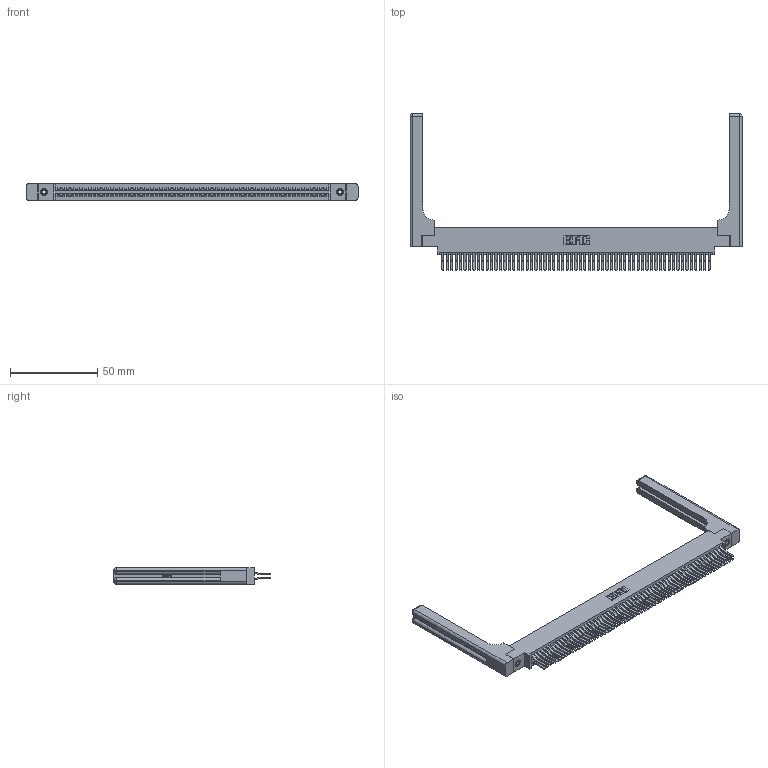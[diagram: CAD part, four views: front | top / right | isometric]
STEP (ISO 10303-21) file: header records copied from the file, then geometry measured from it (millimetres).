
FILE_DESCRIPTION (( 'STEP AP203' ), '1' );
FILE_NAME ('395-122-560-858.STEP', '2019-10-28T09:59:10', ( '' ), ( '' ), 'SwSTEP 2.0', 'SolidWorks 2016', '' );
FILE_SCHEMA (( 'CONFIG_CONTROL_DESIGN' ));
Length unit declared in the file: inch
Products named in the file (5): 345 Part_0.170 Offset - 0.156 Dia-TH; 345-292-001_560 Tail; 345-250-001_345-250-001-102; 345-220-058_345-220-058; 395-122-560-858
Assembly tree (127 placements, depth 2):
  395-122-560-858
    345 Part_0.170 Offset - 0.156 Dia-TH
    345-292-001_560 Tail  x122
    345-250-001_345-250-001-102  x2
    345-220-058_345-220-058  x2
Bounding box: 189.97 x 89.72 x 9.4 mm (x, y, z)
Volume: 27791.3 mm3; surface area: 36179.6 mm2
Topology: 127 solids, 127 shells, 6730 faces, 19929 edges, 13102 vertices
Faces by surface type: plane 4258, cylinder 2412, bspline 36, cone 12, sphere 8, torus 4
Entity records: 50706 total; most frequent: CARTESIAN_POINT 9477, ORIENTED_EDGE 8208, DIRECTION 7268, EDGE_CURVE 4104, VECTOR 3632, LINE 3632, VERTEX_POINT 2726, AXIS2_PLACEMENT_3D 1818
